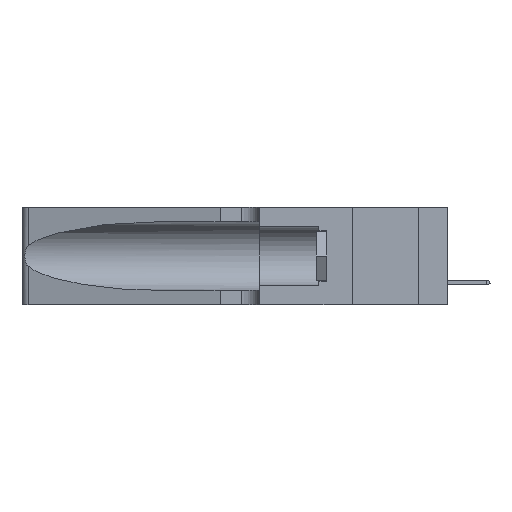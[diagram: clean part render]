
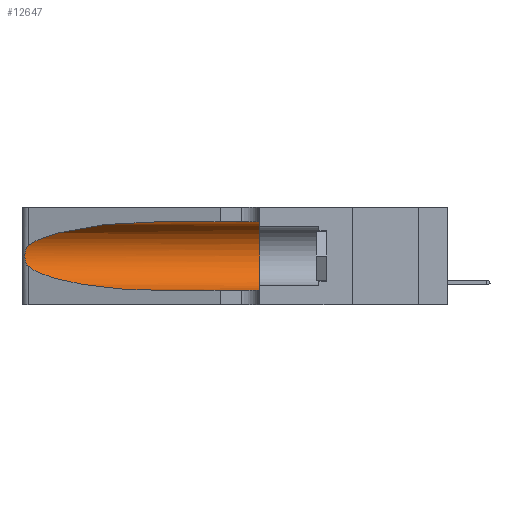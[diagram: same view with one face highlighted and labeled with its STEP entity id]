
A CAD part, left-side view. The second image highlights one B-rep face of the part: STEP entity #12647.
In plain terms, the highlighted cylindrical face has radius 3.308 mm (diameter 6.617 mm), a partial arc.
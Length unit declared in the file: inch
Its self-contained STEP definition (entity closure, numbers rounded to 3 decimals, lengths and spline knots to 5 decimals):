
#211 = CARTESIAN_POINT ( 'NONE',  ( 0.2373, 1.15595, 0.28018 ) ) ;
#348 = CARTESIAN_POINT ( 'NONE',  ( 0.1305, 0.35, 0.31525 ) ) ;
#793 = CARTESIAN_POINT ( 'NONE',  ( 0.1305, 1.61858, 0.05475 ) ) ;
#1541 = EDGE_CURVE ( 'NONE', #16087, #12024, #10613, .T. ) ;
#1911 = ORIENTED_EDGE ( 'NONE', *, *, #12763, .T. ) ;
#2144 = EDGE_LOOP ( 'NONE', ( #25866, #24234, #1911, #16667, #12538, #16303 ) ) ;
#5733 = CARTESIAN_POINT ( 'NONE',  ( 0.1305, 0.35, 0.05475 ) ) ;
#5893 = AXIS2_PLACEMENT_3D ( 'NONE', #18319, #11517, #9503 ) ;
#6095 = CARTESIAN_POINT ( 'NONE',  ( 0.26018, 1.23835, 0.19895 ) ) ;
#6500 = CARTESIAN_POINT ( 'NONE',  ( 0.25555, 1.22993, 0.14849 ) ) ;
#6663 = FACE_OUTER_BOUND ( 'NONE', #2144, .T. ) ;
#7617 = CARTESIAN_POINT ( 'NONE',  ( 0.18966, 0.96281, 0.05475 ) ) ;
#7920 = DIRECTION ( 'NONE',  ( 0., 0., -1. ) ) ;
#7947 = LINE ( 'NONE', #15017, #19032 ) ;
#8077 = CARTESIAN_POINT ( 'NONE',  ( 0.25487, 1.22718, 0.22369 ) ) ;
#8453 = CARTESIAN_POINT ( 'NONE',  ( 0.26075, 1.23896, 0.178 ) ) ;
#8568 = CARTESIAN_POINT ( 'NONE',  ( 0.1305, 1.61858, 0.185 ) ) ;
#8667 = CARTESIAN_POINT ( 'NONE',  ( 0.25639, 1.23186, 0.15144 ) ) ;
#9345 = CARTESIAN_POINT ( 'NONE',  ( 0.1305, 0.72297, 0.31525 ) ) ;
#9503 = DIRECTION ( 'NONE',  ( 0., 0., 1. ) ) ;
#10191 = CARTESIAN_POINT ( 'NONE',  ( 0.25487, 1.22718, 0.14631 ) ) ;
#10613 = CIRCLE ( 'NONE', #5893, 0.13025 ) ;
#11065 = CARTESIAN_POINT ( 'NONE',  ( 0.25487, 1.22718, 0.14631 ) ) ;
#11517 = DIRECTION ( 'NONE',  ( 0., 1., 0. ) ) ;
#12014 = CYLINDRICAL_SURFACE ( 'NONE', #26037, 0.13025 ) ;
#12024 = VERTEX_POINT ( 'NONE', #5733 ) ;
#12313 = CARTESIAN_POINT ( 'NONE',  ( 0.25487, 1.22718, 0.22369 ) ) ;
#12538 = ORIENTED_EDGE ( 'NONE', *, *, #1541, .F. ) ;
#12647 = ADVANCED_FACE ( 'NONE', ( #6663 ), #12014, .F. ) ;
#12763 = EDGE_CURVE ( 'NONE', #27809, #29349, #26246, .T. ) ;
#12982 = CARTESIAN_POINT ( 'NONE',  ( 0.26017, 1.23833, 0.17102 ) ) ;
#15017 = CARTESIAN_POINT ( 'NONE',  ( 0.1305, 1.61858, 0.31525 ) ) ;
#15165 = EDGE_CURVE ( 'NONE', #19684, #16087, #7947, .T. ) ;
#15579 = B_SPLINE_CURVE_WITH_KNOTS ( 'NONE', 3,
 ( #8077, #21865, #19752, #29377, #20149, #6095, #24473, #8453, #12982, #28957, #22055, #8667, #6500, #22266 ),
 .UNSPECIFIED., .F., .F.,
 ( 4, 2, 2, 2, 2, 2, 4 ),
 ( 0., 0.00027, 0.00053, 0.00107, 0.0016, 0.00187, 0.00214 ),
 .UNSPECIFIED. ) ;
#15582 = DIRECTION ( 'NONE',  ( 0., -1., 0. ) ) ;
#16087 = VERTEX_POINT ( 'NONE', #348 ) ;
#16303 = ORIENTED_EDGE ( 'NONE', *, *, #15165, .F. ) ;
#16667 = ORIENTED_EDGE ( 'NONE', *, *, #23839, .T. ) ;
#16716 = VECTOR ( 'NONE', #19081, 39.37008 ) ;
#18319 = CARTESIAN_POINT ( 'NONE',  ( 0.1305, 0.35, 0.185 ) ) ;
#18487 = EDGE_CURVE ( 'NONE', #19684, #19623, #20882, .T. ) ;
#19032 = VECTOR ( 'NONE', #24106, 39.37008 ) ;
#19081 = DIRECTION ( 'NONE',  ( 0., -1., 0. ) ) ;
#19623 = VERTEX_POINT ( 'NONE', #12313 ) ;
#19684 = VERTEX_POINT ( 'NONE', #29082 ) ;
#19752 = CARTESIAN_POINT ( 'NONE',  ( 0.25639, 1.23184, 0.21858 ) ) ;
#20149 = CARTESIAN_POINT ( 'NONE',  ( 0.25854, 1.2359, 0.20912 ) ) ;
#20643 = LINE ( 'NONE', #793, #16716 ) ;
#20834 = CARTESIAN_POINT ( 'NONE',  ( 0.18966, 0.96281, 0.31525 ) ) ;
#20882 =( BOUNDED_CURVE ( )  B_SPLINE_CURVE ( 3, ( #9345, #20834, #211, #21034 ),
 .UNSPECIFIED., .F., .F. ) 
 B_SPLINE_CURVE_WITH_KNOTS ( ( 4, 4 ),
 ( 1.5708, 2.84003 ),
 .UNSPECIFIED. ) 
 CURVE ( )  GEOMETRIC_REPRESENTATION_ITEM ( )  RATIONAL_B_SPLINE_CURVE ( ( 1., 0.87, 0.87, 1. ) ) 
 REPRESENTATION_ITEM ( '' )  );
#21034 = CARTESIAN_POINT ( 'NONE',  ( 0.25487, 1.22718, 0.22369 ) ) ;
#21865 = CARTESIAN_POINT ( 'NONE',  ( 0.25555, 1.22994, 0.2215 ) ) ;
#22055 = CARTESIAN_POINT ( 'NONE',  ( 0.25789, 1.23486, 0.15765 ) ) ;
#22266 = CARTESIAN_POINT ( 'NONE',  ( 0.25487, 1.22718, 0.14631 ) ) ;
#23287 = CARTESIAN_POINT ( 'NONE',  ( 0.1305, 0.72297, 0.05475 ) ) ;
#23607 = CARTESIAN_POINT ( 'NONE',  ( 0.1305, 0.72297, 0.05475 ) ) ;
#23839 = EDGE_CURVE ( 'NONE', #29349, #12024, #20643, .T. ) ;
#24106 = DIRECTION ( 'NONE',  ( 0., -1., 0. ) ) ;
#24234 = ORIENTED_EDGE ( 'NONE', *, *, #25555, .T. ) ;
#24473 = CARTESIAN_POINT ( 'NONE',  ( 0.26075, 1.23896, 0.19203 ) ) ;
#25555 = EDGE_CURVE ( 'NONE', #19623, #27809, #15579, .T. ) ;
#25866 = ORIENTED_EDGE ( 'NONE', *, *, #18487, .T. ) ;
#26037 = AXIS2_PLACEMENT_3D ( 'NONE', #8568, #15582, #7920 ) ;
#26246 =( BOUNDED_CURVE ( )  B_SPLINE_CURVE ( 3, ( #10191, #28096, #7617, #23607 ),
 .UNSPECIFIED., .F., .F. ) 
 B_SPLINE_CURVE_WITH_KNOTS ( ( 4, 4 ),
 ( 3.44316, 4.71239 ),
 .UNSPECIFIED. ) 
 CURVE ( )  GEOMETRIC_REPRESENTATION_ITEM ( )  RATIONAL_B_SPLINE_CURVE ( ( 1., 0.87, 0.87, 1. ) ) 
 REPRESENTATION_ITEM ( '' )  );
#27809 = VERTEX_POINT ( 'NONE', #11065 ) ;
#28096 = CARTESIAN_POINT ( 'NONE',  ( 0.2373, 1.15595, 0.08982 ) ) ;
#28957 = CARTESIAN_POINT ( 'NONE',  ( 0.25856, 1.23593, 0.16098 ) ) ;
#29082 = CARTESIAN_POINT ( 'NONE',  ( 0.1305, 0.72297, 0.31525 ) ) ;
#29349 = VERTEX_POINT ( 'NONE', #23287 ) ;
#29377 = CARTESIAN_POINT ( 'NONE',  ( 0.25787, 1.23484, 0.2124 ) ) ;
